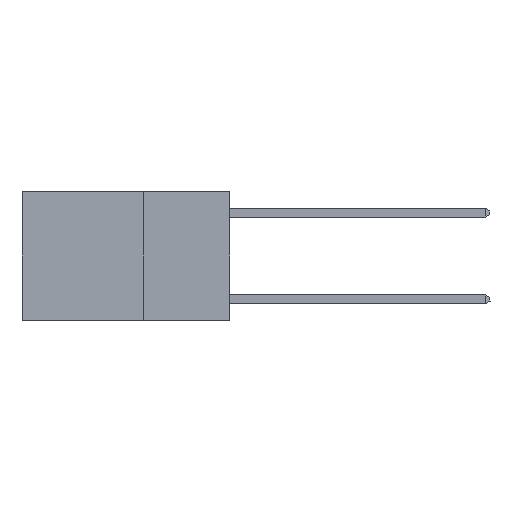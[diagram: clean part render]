
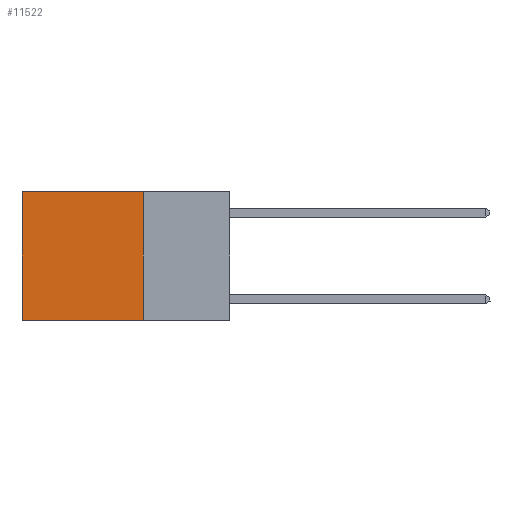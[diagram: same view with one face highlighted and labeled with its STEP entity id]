
A CAD part, left-side view. The second image highlights one B-rep face of the part: STEP entity #11522.
In plain terms, the highlighted planar face has unit normal (-1, 0, 0).
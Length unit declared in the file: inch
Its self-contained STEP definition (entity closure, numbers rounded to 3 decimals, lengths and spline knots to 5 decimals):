
#60 = CARTESIAN_POINT ( 'NONE',  ( 0.2625, 0.6, 0. ) ) ;
#365 = CARTESIAN_POINT ( 'NONE',  ( 0.2625, 0.25, 0. ) ) ;
#1225 = VECTOR ( 'NONE', #10307, 39.37008 ) ;
#1489 = VERTEX_POINT ( 'NONE', #60 ) ;
#1660 = EDGE_CURVE ( 'NONE', #7253, #5876, #6211, .T. ) ;
#1864 = EDGE_CURVE ( 'NONE', #1489, #5876, #11150, .T. ) ;
#1911 = DIRECTION ( 'NONE',  ( 0., 0., -1. ) ) ;
#2216 = EDGE_LOOP ( 'NONE', ( #7489, #8066, #8188, #8217 ) ) ;
#2384 = DIRECTION ( 'NONE',  ( 0., 0., -1. ) ) ;
#2690 = VECTOR ( 'NONE', #9983, 39.37008 ) ;
#2823 = EDGE_CURVE ( 'NONE', #10470, #1489, #3318, .T. ) ;
#2893 = CARTESIAN_POINT ( 'NONE',  ( 0.2625, 0.6, 0. ) ) ;
#3318 = LINE ( 'NONE', #4861, #2690 ) ;
#3995 = FACE_OUTER_BOUND ( 'NONE', #2216, .T. ) ;
#4002 = AXIS2_PLACEMENT_3D ( 'NONE', #365, #7796, #2384 ) ;
#4257 = PLANE ( 'NONE',  #4002 ) ;
#4861 = CARTESIAN_POINT ( 'NONE',  ( 0.2625, 0.25, 0. ) ) ;
#5133 = VECTOR ( 'NONE', #9940, 39.37008 ) ;
#5368 = CARTESIAN_POINT ( 'NONE',  ( 0.2625, 0.25, 0. ) ) ;
#5876 = VERTEX_POINT ( 'NONE', #11405 ) ;
#6154 = CARTESIAN_POINT ( 'NONE',  ( 0.2625, 0.25, -0.37 ) ) ;
#6211 = LINE ( 'NONE', #6154, #1225 ) ;
#6512 = CARTESIAN_POINT ( 'NONE',  ( 0.2625, 0.25, -0.37 ) ) ;
#7253 = VERTEX_POINT ( 'NONE', #6512 ) ;
#7489 = ORIENTED_EDGE ( 'NONE', *, *, #1864, .T. ) ;
#7731 = LINE ( 'NONE', #9132, #5133 ) ;
#7796 = DIRECTION ( 'NONE',  ( 1., 0., 0. ) ) ;
#8066 = ORIENTED_EDGE ( 'NONE', *, *, #1660, .F. ) ;
#8188 = ORIENTED_EDGE ( 'NONE', *, *, #9713, .F. ) ;
#8217 = ORIENTED_EDGE ( 'NONE', *, *, #2823, .T. ) ;
#9132 = CARTESIAN_POINT ( 'NONE',  ( 0.2625, 0.25, 0. ) ) ;
#9713 = EDGE_CURVE ( 'NONE', #10470, #7253, #7731, .T. ) ;
#9940 = DIRECTION ( 'NONE',  ( 0., 0., -1. ) ) ;
#9983 = DIRECTION ( 'NONE',  ( 0., 1., 0. ) ) ;
#10307 = DIRECTION ( 'NONE',  ( 0., 1., 0. ) ) ;
#10470 = VERTEX_POINT ( 'NONE', #5368 ) ;
#10901 = VECTOR ( 'NONE', #1911, 39.37008 ) ;
#11150 = LINE ( 'NONE', #2893, #10901 ) ;
#11405 = CARTESIAN_POINT ( 'NONE',  ( 0.2625, 0.6, -0.37 ) ) ;
#11522 = ADVANCED_FACE ( 'NONE', ( #3995 ), #4257, .F. ) ;
